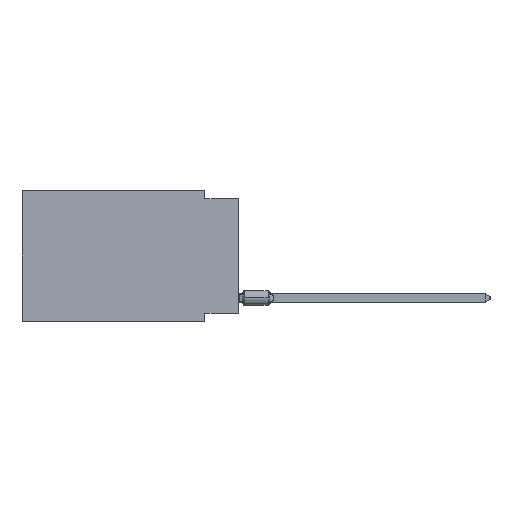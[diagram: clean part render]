
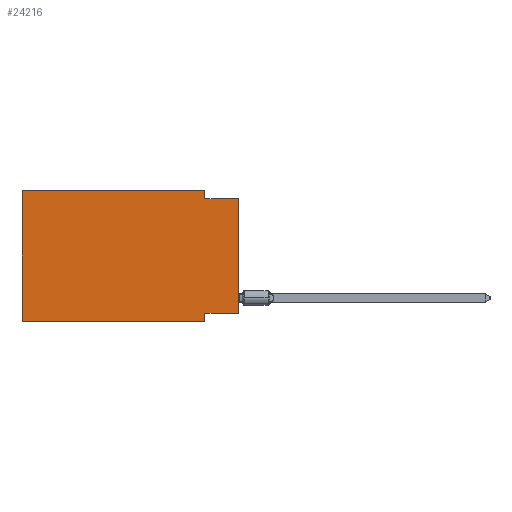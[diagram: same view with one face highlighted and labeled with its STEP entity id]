
A CAD part, left-side view. The second image highlights one B-rep face of the part: STEP entity #24216.
In plain terms, the highlighted planar face has unit normal (-1, 0, 0).
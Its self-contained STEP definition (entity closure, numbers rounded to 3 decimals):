
#1500 = CARTESIAN_POINT ( 'NONE',  ( 0., 0., -0.635 ) ) ;
#5370 = DIRECTION ( 'NONE',  ( 0., 0., -1. ) ) ;
#5775 = EDGE_CURVE ( 'NONE', #74288, #9971, #29496, .T. ) ;
#5798 = LINE ( 'NONE', #64423, #14113 ) ;
#6279 = VECTOR ( 'NONE', #15862, 1000. ) ;
#7752 = VECTOR ( 'NONE', #12656, 1000. ) ;
#7764 = DIRECTION ( 'NONE',  ( 0., -1., 0. ) ) ;
#8164 = LINE ( 'NONE', #54159, #62032 ) ;
#9574 = CARTESIAN_POINT ( 'NONE',  ( 0., 2.54, -0.635 ) ) ;
#9624 = VERTEX_POINT ( 'NONE', #24695 ) ;
#9971 = VERTEX_POINT ( 'NONE', #74870 ) ;
#10427 = EDGE_CURVE ( 'NONE', #69463, #9971, #64753, .T. ) ;
#11183 = DIRECTION ( 'NONE',  ( 0., 0., 1. ) ) ;
#11484 = EDGE_CURVE ( 'NONE', #69463, #9624, #23764, .T. ) ;
#12026 = CARTESIAN_POINT ( 'NONE',  ( 0., 2.54, -9.271 ) ) ;
#12656 = DIRECTION ( 'NONE',  ( 0., -1., 0. ) ) ;
#12868 = ORIENTED_EDGE ( 'NONE', *, *, #34785, .F. ) ;
#14113 = VECTOR ( 'NONE', #11183, 1000. ) ;
#14687 = VERTEX_POINT ( 'NONE', #28096 ) ;
#15276 = VERTEX_POINT ( 'NONE', #1500 ) ;
#15862 = DIRECTION ( 'NONE',  ( 0., 0., -1. ) ) ;
#17202 = EDGE_CURVE ( 'NONE', #14687, #15276, #5798, .T. ) ;
#17594 = DIRECTION ( 'NONE',  ( 0., -1., 0. ) ) ;
#18261 = VECTOR ( 'NONE', #38208, 1000. ) ;
#22239 = CARTESIAN_POINT ( 'NONE',  ( 0., 16.383, 0. ) ) ;
#22684 = EDGE_LOOP ( 'NONE', ( #54637, #71521, #40596, #45493, #26047, #27429, #74048, #12868 ) ) ;
#23764 = LINE ( 'NONE', #75164, #66807 ) ;
#24216 = ADVANCED_FACE ( 'NONE', ( #40603 ), #35215, .F. ) ;
#24695 = CARTESIAN_POINT ( 'NONE',  ( 0., 16.383, 0. ) ) ;
#26047 = ORIENTED_EDGE ( 'NONE', *, *, #11484, .F. ) ;
#27429 = ORIENTED_EDGE ( 'NONE', *, *, #10427, .T. ) ;
#28096 = CARTESIAN_POINT ( 'NONE',  ( 0., 0., -9.271 ) ) ;
#29496 = LINE ( 'NONE', #68362, #6279 ) ;
#30224 = VERTEX_POINT ( 'NONE', #9574 ) ;
#31544 = DIRECTION ( 'NONE',  ( 0., 1., 0. ) ) ;
#34229 = VECTOR ( 'NONE', #7764, 1000. ) ;
#34785 = EDGE_CURVE ( 'NONE', #14687, #74288, #8164, .T. ) ;
#35215 = PLANE ( 'NONE',  #60853 ) ;
#36936 = CARTESIAN_POINT ( 'NONE',  ( 0., 16.383, -9.906 ) ) ;
#37898 = CARTESIAN_POINT ( 'NONE',  ( 0., 2.54, 0. ) ) ;
#38208 = DIRECTION ( 'NONE',  ( 0., 0., -1. ) ) ;
#40596 = ORIENTED_EDGE ( 'NONE', *, *, #55458, .F. ) ;
#40603 = FACE_OUTER_BOUND ( 'NONE', #22684, .T. ) ;
#45493 = ORIENTED_EDGE ( 'NONE', *, *, #55734, .F. ) ;
#45606 = DIRECTION ( 'NONE',  ( 1., 0., 0. ) ) ;
#46752 = DIRECTION ( 'NONE',  ( 0., 0., 1. ) ) ;
#47979 = LINE ( 'NONE', #71763, #34229 ) ;
#52875 = CARTESIAN_POINT ( 'NONE',  ( 0., 16.383, -9.906 ) ) ;
#54159 = CARTESIAN_POINT ( 'NONE',  ( 0., 0., -9.271 ) ) ;
#54637 = ORIENTED_EDGE ( 'NONE', *, *, #17202, .T. ) ;
#55458 = EDGE_CURVE ( 'NONE', #56334, #30224, #72353, .T. ) ;
#55734 = EDGE_CURVE ( 'NONE', #9624, #56334, #47979, .T. ) ;
#56334 = VERTEX_POINT ( 'NONE', #37898 ) ;
#60853 = AXIS2_PLACEMENT_3D ( 'NONE', #22239, #45606, #5370 ) ;
#62032 = VECTOR ( 'NONE', #31544, 1000. ) ;
#63570 = LINE ( 'NONE', #70093, #65050 ) ;
#64423 = CARTESIAN_POINT ( 'NONE',  ( 0., 0., 0. ) ) ;
#64753 = LINE ( 'NONE', #52875, #7752 ) ;
#65050 = VECTOR ( 'NONE', #17594, 1000. ) ;
#66218 = CARTESIAN_POINT ( 'NONE',  ( 0., 2.54, 0. ) ) ;
#66807 = VECTOR ( 'NONE', #46752, 1000. ) ;
#68362 = CARTESIAN_POINT ( 'NONE',  ( 0., 2.54, -9.906 ) ) ;
#69463 = VERTEX_POINT ( 'NONE', #36936 ) ;
#70093 = CARTESIAN_POINT ( 'NONE',  ( 0., 0., -0.635 ) ) ;
#71521 = ORIENTED_EDGE ( 'NONE', *, *, #73945, .F. ) ;
#71763 = CARTESIAN_POINT ( 'NONE',  ( 0., 16.383, 0. ) ) ;
#72353 = LINE ( 'NONE', #66218, #18261 ) ;
#73945 = EDGE_CURVE ( 'NONE', #30224, #15276, #63570, .T. ) ;
#74048 = ORIENTED_EDGE ( 'NONE', *, *, #5775, .F. ) ;
#74288 = VERTEX_POINT ( 'NONE', #12026 ) ;
#74870 = CARTESIAN_POINT ( 'NONE',  ( 0., 2.54, -9.906 ) ) ;
#75164 = CARTESIAN_POINT ( 'NONE',  ( 0., 16.383, 0. ) ) ;
